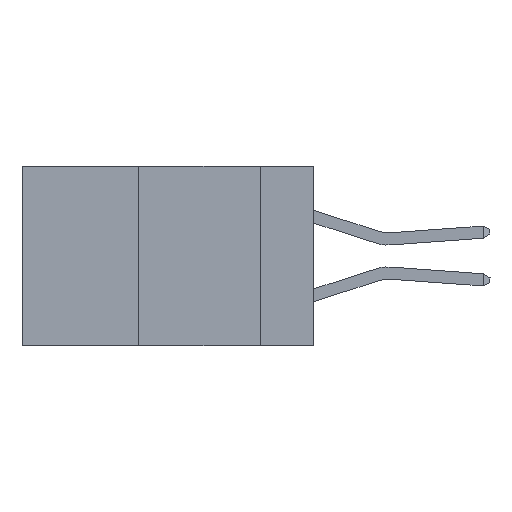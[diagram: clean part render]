
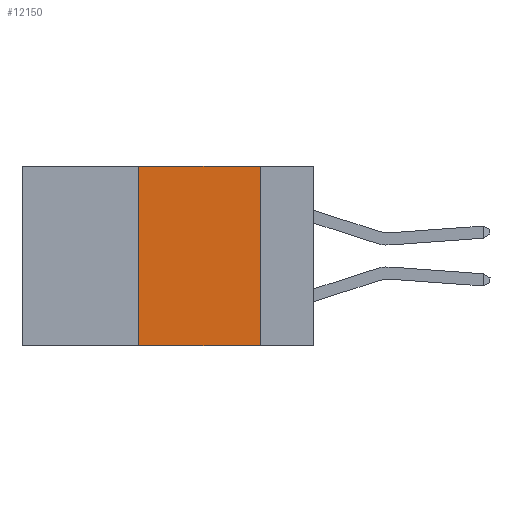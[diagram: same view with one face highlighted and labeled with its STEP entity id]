
A CAD part, left-side view. The second image highlights one B-rep face of the part: STEP entity #12150.
In plain terms, the highlighted planar face has unit normal (-1, 0, 0).
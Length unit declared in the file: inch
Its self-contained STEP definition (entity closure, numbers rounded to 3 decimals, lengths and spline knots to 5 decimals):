
#415 = CARTESIAN_POINT ( 'NONE',  ( 0., 0.36, -0.37 ) ) ;
#559 = ORIENTED_EDGE ( 'NONE', *, *, #5686, .F. ) ;
#602 = PLANE ( 'NONE',  #4367 ) ;
#1333 = DIRECTION ( 'NONE',  ( 0., 0., -1. ) ) ;
#1549 = EDGE_CURVE ( 'NONE', #14003, #12887, #12062, .T. ) ;
#1828 = CARTESIAN_POINT ( 'NONE',  ( 0., 0.6, -0.37 ) ) ;
#2141 = EDGE_CURVE ( 'NONE', #5557, #12887, #5840, .T. ) ;
#2170 = DIRECTION ( 'NONE',  ( 0., -1., 0. ) ) ;
#2624 = CARTESIAN_POINT ( 'NONE',  ( 0., 0.11, 0. ) ) ;
#2705 = CARTESIAN_POINT ( 'NONE',  ( 0., 0.11, 0. ) ) ;
#3057 = CARTESIAN_POINT ( 'NONE',  ( 0., 0.6, 0. ) ) ;
#3424 = CARTESIAN_POINT ( 'NONE',  ( 0., 0.6, 0. ) ) ;
#3659 = VECTOR ( 'NONE', #7893, 39.37008 ) ;
#3973 = CARTESIAN_POINT ( 'NONE',  ( 0., 0.36, 0. ) ) ;
#4352 = FACE_OUTER_BOUND ( 'NONE', #7502, .T. ) ;
#4367 = AXIS2_PLACEMENT_3D ( 'NONE', #3424, #12431, #4735 ) ;
#4735 = DIRECTION ( 'NONE',  ( 0., 0., -1. ) ) ;
#4872 = ORIENTED_EDGE ( 'NONE', *, *, #11174, .F. ) ;
#5240 = VECTOR ( 'NONE', #6323, 39.37008 ) ;
#5557 = VERTEX_POINT ( 'NONE', #2705 ) ;
#5686 = EDGE_CURVE ( 'NONE', #13790, #5557, #6303, .T. ) ;
#5840 = LINE ( 'NONE', #2624, #12239 ) ;
#6120 = VECTOR ( 'NONE', #2170, 39.37008 ) ;
#6303 = LINE ( 'NONE', #3057, #6120 ) ;
#6323 = DIRECTION ( 'NONE',  ( 0., -1., 0. ) ) ;
#6710 = ORIENTED_EDGE ( 'NONE', *, *, #2141, .F. ) ;
#6762 = CARTESIAN_POINT ( 'NONE',  ( 0., 0.36, 0. ) ) ;
#7151 = LINE ( 'NONE', #3973, #3659 ) ;
#7502 = EDGE_LOOP ( 'NONE', ( #6710, #559, #4872, #10815 ) ) ;
#7893 = DIRECTION ( 'NONE',  ( 0., 0., 1. ) ) ;
#10815 = ORIENTED_EDGE ( 'NONE', *, *, #1549, .T. ) ;
#11174 = EDGE_CURVE ( 'NONE', #14003, #13790, #7151, .T. ) ;
#12062 = LINE ( 'NONE', #1828, #5240 ) ;
#12150 = ADVANCED_FACE ( 'NONE', ( #4352 ), #602, .F. ) ;
#12239 = VECTOR ( 'NONE', #1333, 39.37008 ) ;
#12431 = DIRECTION ( 'NONE',  ( 1., 0., 0. ) ) ;
#12887 = VERTEX_POINT ( 'NONE', #15160 ) ;
#13790 = VERTEX_POINT ( 'NONE', #6762 ) ;
#14003 = VERTEX_POINT ( 'NONE', #415 ) ;
#15160 = CARTESIAN_POINT ( 'NONE',  ( 0., 0.11, -0.37 ) ) ;
